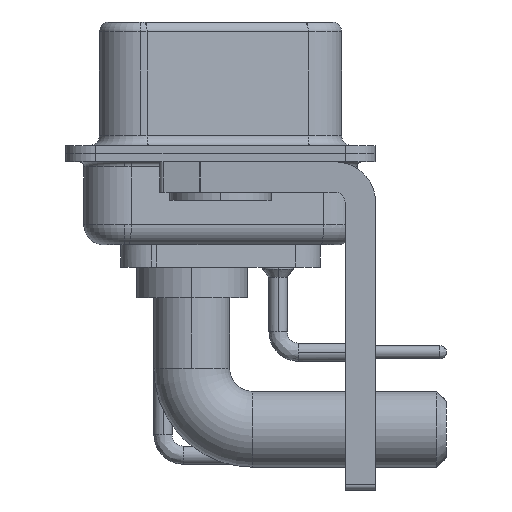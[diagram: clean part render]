
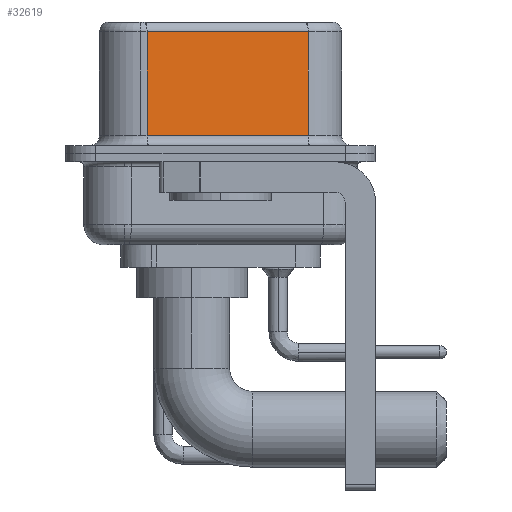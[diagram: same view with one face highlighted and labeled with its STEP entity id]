
A CAD part, left-side view. The second image highlights one B-rep face of the part: STEP entity #32619.
In plain terms, the highlighted planar face has unit normal (-0.985, -0.174, 0).
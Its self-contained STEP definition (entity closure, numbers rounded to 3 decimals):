
#436 = CARTESIAN_POINT ( 'NONE',  ( 3.73, 3.628, 6.02 ) ) ;
#864 = FACE_OUTER_BOUND ( 'NONE', #23151, .T. ) ;
#1422 = LINE ( 'NONE', #26391, #15928 ) ;
#2109 = CARTESIAN_POINT ( 'NONE',  ( 5.132, -4.322, 6.02 ) ) ;
#2116 = DIRECTION ( 'NONE',  ( 0., 0., -1. ) ) ;
#3375 = VECTOR ( 'NONE', #31535, 1000. ) ;
#4240 = ORIENTED_EDGE ( 'NONE', *, *, #8313, .F. ) ;
#4453 = CARTESIAN_POINT ( 'NONE',  ( 5.132, -4.322, 0.9 ) ) ;
#4798 = LINE ( 'NONE', #4453, #14287 ) ;
#6147 = VERTEX_POINT ( 'NONE', #10717 ) ;
#7635 = LINE ( 'NONE', #23749, #3375 ) ;
#8313 = EDGE_CURVE ( 'NONE', #12023, #6147, #23213, .T. ) ;
#10443 = EDGE_CURVE ( 'NONE', #31857, #6147, #4798, .T. ) ;
#10717 = CARTESIAN_POINT ( 'NONE',  ( 5.132, -4.322, 0.9 ) ) ;
#11445 = ORIENTED_EDGE ( 'NONE', *, *, #25352, .T. ) ;
#12023 = VERTEX_POINT ( 'NONE', #2109 ) ;
#12251 = DIRECTION ( 'NONE',  ( -0.174, 0.985, 0. ) ) ;
#12936 = CARTESIAN_POINT ( 'NONE',  ( 5.132, -4.322, 6.52 ) ) ;
#14287 = VECTOR ( 'NONE', #20773, 1000. ) ;
#15528 = ORIENTED_EDGE ( 'NONE', *, *, #28641, .T. ) ;
#15928 = VECTOR ( 'NONE', #12251, 1000. ) ;
#16485 = DIRECTION ( 'NONE',  ( 0.985, 0.174, 0. ) ) ;
#20773 = DIRECTION ( 'NONE',  ( 0.174, -0.985, 0. ) ) ;
#21987 = PLANE ( 'NONE',  #23942 ) ;
#22159 = CARTESIAN_POINT ( 'NONE',  ( 5.132, -4.322, 6.52 ) ) ;
#23151 = EDGE_LOOP ( 'NONE', ( #4240, #11445, #15528, #24920 ) ) ;
#23213 = LINE ( 'NONE', #12936, #34492 ) ;
#23749 = CARTESIAN_POINT ( 'NONE',  ( 3.73, 3.628, 6.52 ) ) ;
#23942 = AXIS2_PLACEMENT_3D ( 'NONE', #22159, #16485, #27289 ) ;
#23962 = CARTESIAN_POINT ( 'NONE',  ( 3.73, 3.628, 0.9 ) ) ;
#24920 = ORIENTED_EDGE ( 'NONE', *, *, #10443, .T. ) ;
#25352 = EDGE_CURVE ( 'NONE', #12023, #30307, #1422, .T. ) ;
#26391 = CARTESIAN_POINT ( 'NONE',  ( 5.132, -4.322, 6.02 ) ) ;
#27289 = DIRECTION ( 'NONE',  ( -0.174, 0.985, 0. ) ) ;
#28641 = EDGE_CURVE ( 'NONE', #30307, #31857, #7635, .T. ) ;
#30307 = VERTEX_POINT ( 'NONE', #436 ) ;
#31535 = DIRECTION ( 'NONE',  ( 0., 0., -1. ) ) ;
#31857 = VERTEX_POINT ( 'NONE', #23962 ) ;
#32619 = ADVANCED_FACE ( 'NONE', ( #864 ), #21987, .F. ) ;
#34492 = VECTOR ( 'NONE', #2116, 1000. ) ;
